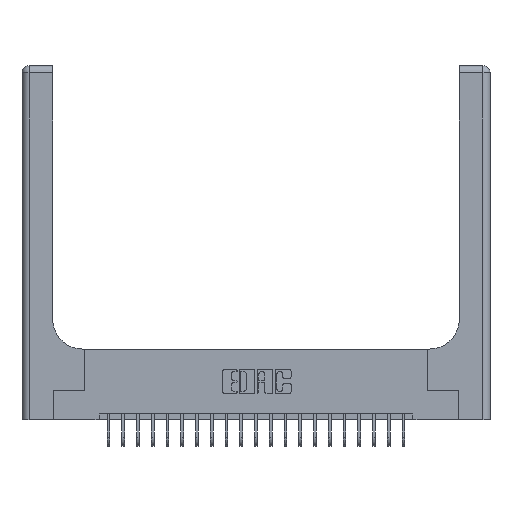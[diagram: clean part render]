
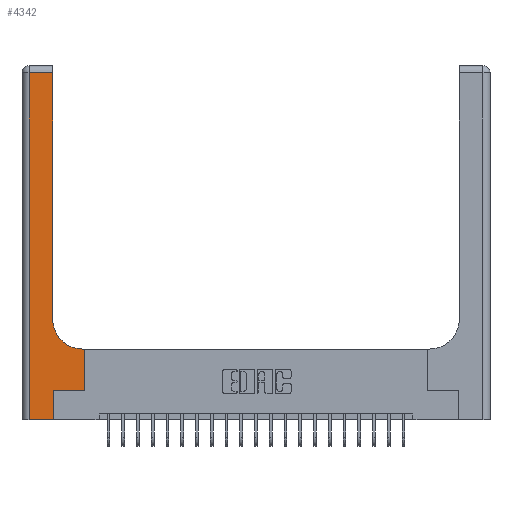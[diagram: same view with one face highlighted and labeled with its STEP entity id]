
A CAD part, top view. The second image highlights one B-rep face of the part: STEP entity #4342.
In plain terms, the highlighted planar face has unit normal (0, 0, 1).
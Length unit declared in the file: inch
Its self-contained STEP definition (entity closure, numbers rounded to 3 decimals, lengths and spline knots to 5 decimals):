
#84 = EDGE_CURVE ( 'NONE', #2176, #2423, #18634, .T. ) ;
#292 = VECTOR ( 'NONE', #19531, 39.37008 ) ;
#803 = DIRECTION ( 'NONE',  ( 0., 1., 0. ) ) ;
#1101 = ORIENTED_EDGE ( 'NONE', *, *, #9984, .T. ) ;
#1544 = CARTESIAN_POINT ( 'NONE',  ( 0.26, 2.94, 0.37 ) ) ;
#1993 = ORIENTED_EDGE ( 'NONE', *, *, #2989, .T. ) ;
#2116 = VERTEX_POINT ( 'NONE', #20136 ) ;
#2176 = VERTEX_POINT ( 'NONE', #9637 ) ;
#2423 = VERTEX_POINT ( 'NONE', #5049 ) ;
#2955 = EDGE_CURVE ( 'NONE', #11943, #23238, #22469, .T. ) ;
#2989 = EDGE_CURVE ( 'NONE', #22063, #2116, #14555, .T. ) ;
#3034 = AXIS2_PLACEMENT_3D ( 'NONE', #13538, #6298, #18940 ) ;
#3215 = EDGE_CURVE ( 'NONE', #23238, #22063, #9406, .T. ) ;
#3301 = EDGE_CURVE ( 'NONE', #2423, #11167, #23325, .T. ) ;
#3554 = ORIENTED_EDGE ( 'NONE', *, *, #8390, .T. ) ;
#4156 = CARTESIAN_POINT ( 'NONE',  ( 0., 3., 0.37 ) ) ;
#4276 = CARTESIAN_POINT ( 'NONE',  ( 0.528, 0.6, 0.37 ) ) ;
#4342 = ADVANCED_FACE ( 'NONE', ( #18669 ), #18456, .F. ) ;
#4470 = VERTEX_POINT ( 'NONE', #4805 ) ;
#4500 = CARTESIAN_POINT ( 'NONE',  ( 0.265, 0., 0.37 ) ) ;
#4805 = CARTESIAN_POINT ( 'NONE',  ( 0.51, 0.6, 0.37 ) ) ;
#5049 = CARTESIAN_POINT ( 'NONE',  ( 0.528, 0.25, 0.37 ) ) ;
#5173 = LINE ( 'NONE', #23152, #292 ) ;
#5969 = DIRECTION ( 'NONE',  ( -1., 0., 0. ) ) ;
#6298 = DIRECTION ( 'NONE',  ( 0., 0., -1. ) ) ;
#6549 = EDGE_LOOP ( 'NONE', ( #22590, #7748, #21346, #1993, #10741, #15394, #13035, #3554, #1101 ) ) ;
#7141 = VECTOR ( 'NONE', #18061, 39.37008 ) ;
#7400 = CARTESIAN_POINT ( 'NONE',  ( 0.26, 0.85, 0.37 ) ) ;
#7716 = VECTOR ( 'NONE', #20948, 39.37008 ) ;
#7748 = ORIENTED_EDGE ( 'NONE', *, *, #2955, .T. ) ;
#8122 = DIRECTION ( 'NONE',  ( -1., 0., 0. ) ) ;
#8390 = EDGE_CURVE ( 'NONE', #11167, #4470, #5173, .T. ) ;
#8668 = CARTESIAN_POINT ( 'NONE',  ( 0.06, 2.94, 0.37 ) ) ;
#8930 = CARTESIAN_POINT ( 'NONE',  ( 0.06, 3., 0.37 ) ) ;
#9279 = CARTESIAN_POINT ( 'NONE',  ( 0.528, 0.25, 0.37 ) ) ;
#9406 = LINE ( 'NONE', #8930, #7141 ) ;
#9637 = CARTESIAN_POINT ( 'NONE',  ( 0.265, 0.25, 0.37 ) ) ;
#9984 = EDGE_CURVE ( 'NONE', #4470, #22775, #12507, .T. ) ;
#10741 = ORIENTED_EDGE ( 'NONE', *, *, #17249, .T. ) ;
#11167 = VERTEX_POINT ( 'NONE', #4276 ) ;
#11943 = VERTEX_POINT ( 'NONE', #1544 ) ;
#12355 = EDGE_CURVE ( 'NONE', #22775, #11943, #21113, .T. ) ;
#12507 = CIRCLE ( 'NONE', #3034, 0.25 ) ;
#13035 = ORIENTED_EDGE ( 'NONE', *, *, #3301, .T. ) ;
#13264 = DIRECTION ( 'NONE',  ( 0., 1., 0. ) ) ;
#13538 = CARTESIAN_POINT ( 'NONE',  ( 0.51, 0.85, 0.37 ) ) ;
#13619 = CARTESIAN_POINT ( 'NONE',  ( 0., 0., 0.37 ) ) ;
#13818 = VECTOR ( 'NONE', #22879, 39.37008 ) ;
#14166 = CARTESIAN_POINT ( 'NONE',  ( 0.06, 0., 0.37 ) ) ;
#14555 = LINE ( 'NONE', #13619, #16837 ) ;
#15394 = ORIENTED_EDGE ( 'NONE', *, *, #84, .T. ) ;
#16250 = VECTOR ( 'NONE', #13264, 39.37008 ) ;
#16837 = VECTOR ( 'NONE', #19252, 39.37008 ) ;
#16874 = DIRECTION ( 'NONE',  ( 0., 0., -1. ) ) ;
#17249 = EDGE_CURVE ( 'NONE', #2116, #2176, #23404, .T. ) ;
#17453 = CARTESIAN_POINT ( 'NONE',  ( 0.26, 3., 0.37 ) ) ;
#17461 = CARTESIAN_POINT ( 'NONE',  ( 0.265, 0.25, 0.37 ) ) ;
#18061 = DIRECTION ( 'NONE',  ( 0., -1., 0. ) ) ;
#18456 = PLANE ( 'NONE',  #22092 ) ;
#18634 = LINE ( 'NONE', #17461, #13818 ) ;
#18669 = FACE_OUTER_BOUND ( 'NONE', #6549, .T. ) ;
#18940 = DIRECTION ( 'NONE',  ( 1., 0., 0. ) ) ;
#19189 = VECTOR ( 'NONE', #803, 39.37008 ) ;
#19252 = DIRECTION ( 'NONE',  ( 1., 0., 0. ) ) ;
#19531 = DIRECTION ( 'NONE',  ( -1., 0., 0. ) ) ;
#20136 = CARTESIAN_POINT ( 'NONE',  ( 0.265, 0., 0.37 ) ) ;
#20948 = DIRECTION ( 'NONE',  ( 0., 1., 0. ) ) ;
#21113 = LINE ( 'NONE', #17453, #7716 ) ;
#21184 = CARTESIAN_POINT ( 'NONE',  ( 0., 2.94, 0.37 ) ) ;
#21346 = ORIENTED_EDGE ( 'NONE', *, *, #3215, .T. ) ;
#21655 = VECTOR ( 'NONE', #8122, 39.37008 ) ;
#22063 = VERTEX_POINT ( 'NONE', #14166 ) ;
#22092 = AXIS2_PLACEMENT_3D ( 'NONE', #4156, #16874, #5969 ) ;
#22469 = LINE ( 'NONE', #21184, #21655 ) ;
#22590 = ORIENTED_EDGE ( 'NONE', *, *, #12355, .T. ) ;
#22775 = VERTEX_POINT ( 'NONE', #7400 ) ;
#22879 = DIRECTION ( 'NONE',  ( 1., 0., 0. ) ) ;
#23152 = CARTESIAN_POINT ( 'NONE',  ( 0.26, 0.6, 0.37 ) ) ;
#23238 = VERTEX_POINT ( 'NONE', #8668 ) ;
#23325 = LINE ( 'NONE', #9279, #16250 ) ;
#23404 = LINE ( 'NONE', #4500, #19189 ) ;
